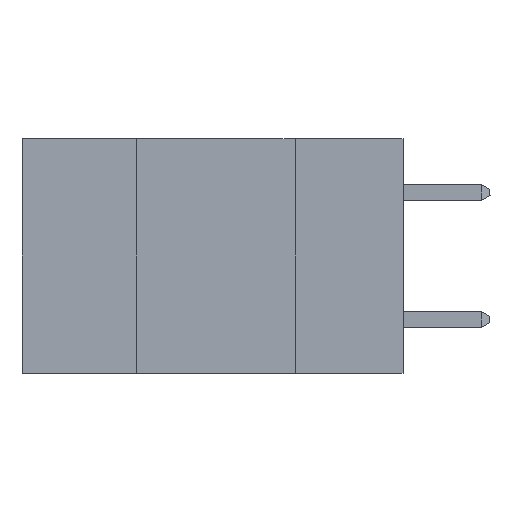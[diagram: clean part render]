
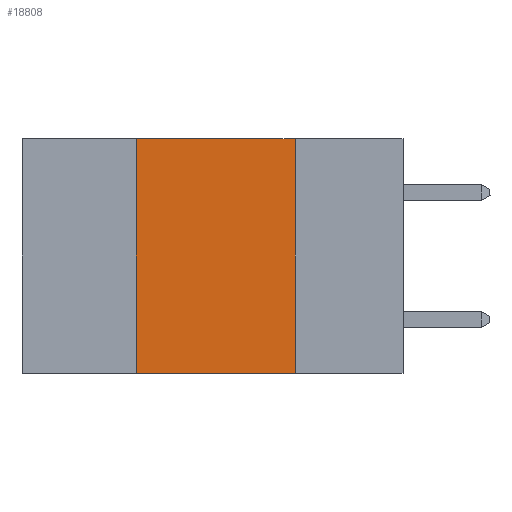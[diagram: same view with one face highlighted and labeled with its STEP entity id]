
A CAD part, left-side view. The second image highlights one B-rep face of the part: STEP entity #18808.
In plain terms, the highlighted planar face has unit normal (-1, 0, 0).
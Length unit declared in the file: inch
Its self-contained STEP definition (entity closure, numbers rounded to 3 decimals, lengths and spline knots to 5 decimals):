
#951 = EDGE_CURVE ( 'NONE', #10323, #19816, #11162, .T. ) ;
#1532 = CARTESIAN_POINT ( 'NONE',  ( 0., 0.17, 0. ) ) ;
#1718 = EDGE_CURVE ( 'NONE', #6591, #16301, #11067, .T. ) ;
#3659 = DIRECTION ( 'NONE',  ( 0., 0., -1. ) ) ;
#4274 = AXIS2_PLACEMENT_3D ( 'NONE', #13278, #7441, #3659 ) ;
#4860 = CARTESIAN_POINT ( 'NONE',  ( 0., 0.6, 0. ) ) ;
#5749 = PLANE ( 'NONE',  #4274 ) ;
#6284 = VECTOR ( 'NONE', #12781, 39.37008 ) ;
#6316 = LINE ( 'NONE', #24402, #22583 ) ;
#6591 = VERTEX_POINT ( 'NONE', #19293 ) ;
#7441 = DIRECTION ( 'NONE',  ( 1., 0., 0. ) ) ;
#8514 = CARTESIAN_POINT ( 'NONE',  ( 0., 0.42, 0. ) ) ;
#8785 = EDGE_CURVE ( 'NONE', #16301, #10323, #16550, .T. ) ;
#9984 = ORIENTED_EDGE ( 'NONE', *, *, #1718, .F. ) ;
#10323 = VERTEX_POINT ( 'NONE', #15880 ) ;
#11067 = LINE ( 'NONE', #8514, #16366 ) ;
#11162 = LINE ( 'NONE', #1532, #23494 ) ;
#12463 = ORIENTED_EDGE ( 'NONE', *, *, #8785, .F. ) ;
#12781 = DIRECTION ( 'NONE',  ( 0., -1., 0. ) ) ;
#13278 = CARTESIAN_POINT ( 'NONE',  ( 0., 0.6, 0. ) ) ;
#13481 = DIRECTION ( 'NONE',  ( 0., 0., -1. ) ) ;
#13771 = CARTESIAN_POINT ( 'NONE',  ( 0., 0.42, 0. ) ) ;
#15880 = CARTESIAN_POINT ( 'NONE',  ( 0., 0.17, 0. ) ) ;
#16301 = VERTEX_POINT ( 'NONE', #13771 ) ;
#16366 = VECTOR ( 'NONE', #18862, 39.37008 ) ;
#16550 = LINE ( 'NONE', #4860, #6284 ) ;
#17051 = ORIENTED_EDGE ( 'NONE', *, *, #19986, .T. ) ;
#18808 = ADVANCED_FACE ( 'NONE', ( #21096 ), #5749, .F. ) ;
#18862 = DIRECTION ( 'NONE',  ( 0., 0., 1. ) ) ;
#19293 = CARTESIAN_POINT ( 'NONE',  ( 0., 0.42, -0.37 ) ) ;
#19408 = ORIENTED_EDGE ( 'NONE', *, *, #951, .F. ) ;
#19816 = VERTEX_POINT ( 'NONE', #19976 ) ;
#19976 = CARTESIAN_POINT ( 'NONE',  ( 0., 0.17, -0.37 ) ) ;
#19986 = EDGE_CURVE ( 'NONE', #6591, #19816, #6316, .T. ) ;
#20095 = DIRECTION ( 'NONE',  ( 0., -1., 0. ) ) ;
#21096 = FACE_OUTER_BOUND ( 'NONE', #23900, .T. ) ;
#22583 = VECTOR ( 'NONE', #20095, 39.37008 ) ;
#23494 = VECTOR ( 'NONE', #13481, 39.37008 ) ;
#23900 = EDGE_LOOP ( 'NONE', ( #19408, #12463, #9984, #17051 ) ) ;
#24402 = CARTESIAN_POINT ( 'NONE',  ( 0., 0.6, -0.37 ) ) ;
